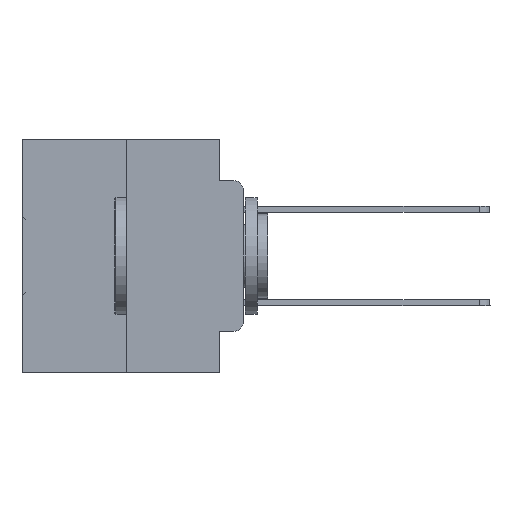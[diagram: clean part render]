
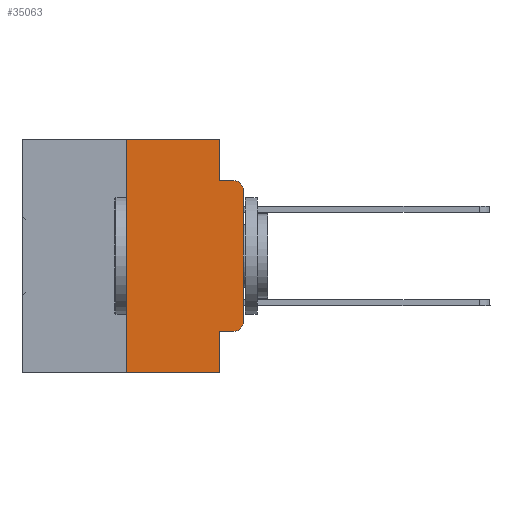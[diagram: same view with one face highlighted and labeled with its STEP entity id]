
A CAD part, left-side view. The second image highlights one B-rep face of the part: STEP entity #35063.
In plain terms, the highlighted planar face has unit normal (-1, 0, 0).
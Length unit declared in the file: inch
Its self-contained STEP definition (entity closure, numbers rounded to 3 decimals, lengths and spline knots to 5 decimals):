
#1004 = CARTESIAN_POINT ( 'NONE',  ( 0., 0.473, 0. ) ) ;
#1173 = VERTEX_POINT ( 'NONE', #15006 ) ;
#1359 = VERTEX_POINT ( 'NONE', #16449 ) ;
#1741 = ORIENTED_EDGE ( 'NONE', *, *, #24701, .F. ) ;
#1871 = EDGE_CURVE ( 'NONE', #1359, #23821, #35806, .T. ) ;
#2392 = CARTESIAN_POINT ( 'NONE',  ( 0., 0.473, -0.5 ) ) ;
#2427 = VECTOR ( 'NONE', #19579, 39.37008 ) ;
#2943 = VERTEX_POINT ( 'NONE', #32973 ) ;
#2980 = DIRECTION ( 'NONE',  ( 0., -1., 0. ) ) ;
#3406 = VECTOR ( 'NONE', #5898, 39.37008 ) ;
#3956 = CARTESIAN_POINT ( 'NONE',  ( 0., 0.051, 0. ) ) ;
#4497 = LINE ( 'NONE', #15174, #22617 ) ;
#4695 = CARTESIAN_POINT ( 'NONE',  ( 0., 0.02, -0.0885 ) ) ;
#5161 = LINE ( 'NONE', #36146, #30850 ) ;
#5889 = VECTOR ( 'NONE', #12418, 39.37008 ) ;
#5898 = DIRECTION ( 'NONE',  ( 0., -1., 0. ) ) ;
#6223 = ORIENTED_EDGE ( 'NONE', *, *, #7106, .F. ) ;
#6563 = DIRECTION ( 'NONE',  ( 0., 0., 1. ) ) ;
#6606 = LINE ( 'NONE', #1004, #5889 ) ;
#7106 = EDGE_CURVE ( 'NONE', #32539, #14597, #28171, .T. ) ;
#7516 = EDGE_CURVE ( 'NONE', #1359, #24242, #30748, .T. ) ;
#8581 = DIRECTION ( 'NONE',  ( 0., 0., -1. ) ) ;
#8769 = CARTESIAN_POINT ( 'NONE',  ( 0., 0.051, 0. ) ) ;
#9318 = CARTESIAN_POINT ( 'NONE',  ( 0., 0.02, -0.1085 ) ) ;
#10824 = AXIS2_PLACEMENT_3D ( 'NONE', #9318, #17903, #11749 ) ;
#11371 = EDGE_CURVE ( 'NONE', #18993, #2943, #5161, .T. ) ;
#11749 = DIRECTION ( 'NONE',  ( 0., 0., -1. ) ) ;
#11957 = CARTESIAN_POINT ( 'NONE',  ( 0., 0.051, -0.0885 ) ) ;
#12002 = CARTESIAN_POINT ( 'NONE',  ( 0., 0.02, -0.4115 ) ) ;
#12245 = VECTOR ( 'NONE', #34792, 39.37008 ) ;
#12418 = DIRECTION ( 'NONE',  ( 0., -1., 0. ) ) ;
#13612 = CARTESIAN_POINT ( 'NONE',  ( 0., 0.051, 0. ) ) ;
#14494 = CARTESIAN_POINT ( 'NONE',  ( 0., 0.051, -0.5 ) ) ;
#14597 = VERTEX_POINT ( 'NONE', #28511 ) ;
#15006 = CARTESIAN_POINT ( 'NONE',  ( 0., 0., -0.1085 ) ) ;
#15174 = CARTESIAN_POINT ( 'NONE',  ( 0., 0., 0. ) ) ;
#16449 = CARTESIAN_POINT ( 'NONE',  ( 0., 0.051, -0.4115 ) ) ;
#17198 = CARTESIAN_POINT ( 'NONE',  ( 0., 0., -0.3915 ) ) ;
#17506 = LINE ( 'NONE', #2392, #3406 ) ;
#17903 = DIRECTION ( 'NONE',  ( -1., 0., 0. ) ) ;
#18212 = ORIENTED_EDGE ( 'NONE', *, *, #32080, .F. ) ;
#18993 = VERTEX_POINT ( 'NONE', #35758 ) ;
#19579 = DIRECTION ( 'NONE',  ( 0., 0., -1. ) ) ;
#19903 = CARTESIAN_POINT ( 'NONE',  ( 0., 0.473, 0. ) ) ;
#20169 = ORIENTED_EDGE ( 'NONE', *, *, #7516, .T. ) ;
#20253 = VECTOR ( 'NONE', #2980, 39.37008 ) ;
#20846 = ORIENTED_EDGE ( 'NONE', *, *, #24361, .T. ) ;
#20883 = AXIS2_PLACEMENT_3D ( 'NONE', #19903, #31854, #34648 ) ;
#22328 = VECTOR ( 'NONE', #8581, 39.37008 ) ;
#22404 = EDGE_CURVE ( 'NONE', #18993, #23821, #17506, .T. ) ;
#22617 = VECTOR ( 'NONE', #6563, 39.37008 ) ;
#23158 = AXIS2_PLACEMENT_3D ( 'NONE', #34232, #31801, #23406 ) ;
#23406 = DIRECTION ( 'NONE',  ( 0., 0., -1. ) ) ;
#23821 = VERTEX_POINT ( 'NONE', #14494 ) ;
#24242 = VERTEX_POINT ( 'NONE', #12002 ) ;
#24361 = EDGE_CURVE ( 'NONE', #32962, #1173, #4497, .T. ) ;
#24701 = EDGE_CURVE ( 'NONE', #14597, #28836, #28565, .T. ) ;
#24769 = FACE_OUTER_BOUND ( 'NONE', #34019, .T. ) ;
#25881 = PLANE ( 'NONE',  #20883 ) ;
#25911 = ORIENTED_EDGE ( 'NONE', *, *, #1871, .F. ) ;
#26926 = CIRCLE ( 'NONE', #10824, 0.02 ) ;
#28171 = LINE ( 'NONE', #8769, #22328 ) ;
#28511 = CARTESIAN_POINT ( 'NONE',  ( 0., 0.051, -0.0885 ) ) ;
#28565 = LINE ( 'NONE', #11957, #20253 ) ;
#28836 = VERTEX_POINT ( 'NONE', #4695 ) ;
#30748 = LINE ( 'NONE', #31993, #12245 ) ;
#30850 = VECTOR ( 'NONE', #33931, 39.37008 ) ;
#31801 = DIRECTION ( 'NONE',  ( -1., 0., 0. ) ) ;
#31854 = DIRECTION ( 'NONE',  ( 1., 0., 0. ) ) ;
#31993 = CARTESIAN_POINT ( 'NONE',  ( 0., 0.051, -0.4115 ) ) ;
#32080 = EDGE_CURVE ( 'NONE', #2943, #32539, #6606, .T. ) ;
#32202 = ORIENTED_EDGE ( 'NONE', *, *, #22404, .T. ) ;
#32448 = EDGE_CURVE ( 'NONE', #24242, #32962, #36299, .T. ) ;
#32509 = ORIENTED_EDGE ( 'NONE', *, *, #11371, .F. ) ;
#32539 = VERTEX_POINT ( 'NONE', #3956 ) ;
#32962 = VERTEX_POINT ( 'NONE', #17198 ) ;
#32973 = CARTESIAN_POINT ( 'NONE',  ( 0., 0.25, 0. ) ) ;
#33691 = ORIENTED_EDGE ( 'NONE', *, *, #36505, .T. ) ;
#33931 = DIRECTION ( 'NONE',  ( 0., 0., 1. ) ) ;
#34019 = EDGE_LOOP ( 'NONE', ( #20846, #33691, #1741, #6223, #18212, #32509, #32202, #25911, #20169, #34834 ) ) ;
#34232 = CARTESIAN_POINT ( 'NONE',  ( 0., 0.02, -0.3915 ) ) ;
#34648 = DIRECTION ( 'NONE',  ( 0., 0., -1. ) ) ;
#34792 = DIRECTION ( 'NONE',  ( 0., -1., 0. ) ) ;
#34834 = ORIENTED_EDGE ( 'NONE', *, *, #32448, .T. ) ;
#35063 = ADVANCED_FACE ( 'NONE', ( #24769 ), #25881, .F. ) ;
#35758 = CARTESIAN_POINT ( 'NONE',  ( 0., 0.25, -0.5 ) ) ;
#35806 = LINE ( 'NONE', #13612, #2427 ) ;
#36146 = CARTESIAN_POINT ( 'NONE',  ( 0., 0.25, 0. ) ) ;
#36299 = CIRCLE ( 'NONE', #23158, 0.02 ) ;
#36505 = EDGE_CURVE ( 'NONE', #1173, #28836, #26926, .T. ) ;
